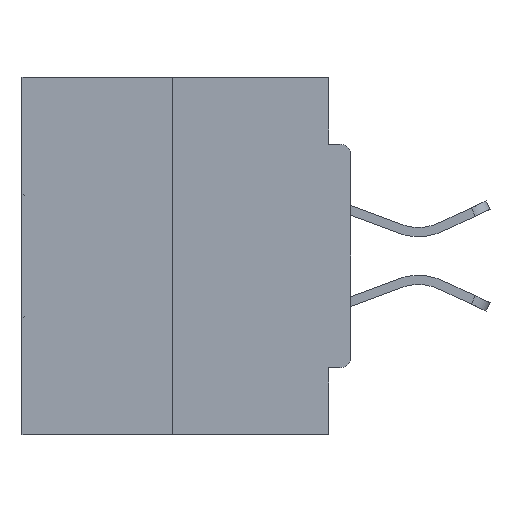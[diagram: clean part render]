
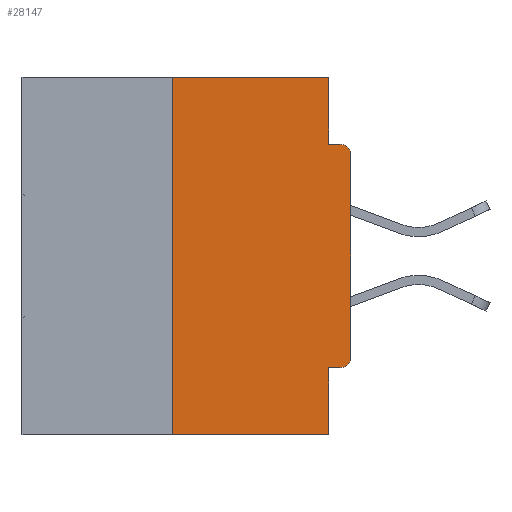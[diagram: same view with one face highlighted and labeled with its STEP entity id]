
A CAD part, left-side view. The second image highlights one B-rep face of the part: STEP entity #28147.
In plain terms, the highlighted planar face has unit normal (-1, 0, 0).
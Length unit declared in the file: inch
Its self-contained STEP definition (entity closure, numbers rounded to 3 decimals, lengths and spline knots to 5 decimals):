
#302 = EDGE_CURVE ( 'NONE', #27543, #3065, #4246, .T. ) ;
#587 = CARTESIAN_POINT ( 'NONE',  ( 0., 0.031, -0.5 ) ) ;
#1290 = CARTESIAN_POINT ( 'NONE',  ( 0., 0.015, -0.1085 ) ) ;
#1628 = DIRECTION ( 'NONE',  ( 1., 0., 0. ) ) ;
#2584 = CARTESIAN_POINT ( 'NONE',  ( 0., 0.25, 0. ) ) ;
#2604 = DIRECTION ( 'NONE',  ( 0., 0., -1. ) ) ;
#2662 = EDGE_CURVE ( 'NONE', #27543, #30808, #4565, .T. ) ;
#3065 = VERTEX_POINT ( 'NONE', #35761 ) ;
#3363 = VECTOR ( 'NONE', #21606, 39.37008 ) ;
#3924 = VECTOR ( 'NONE', #36852, 39.37008 ) ;
#3927 = ORIENTED_EDGE ( 'NONE', *, *, #38037, .F. ) ;
#3954 = ORIENTED_EDGE ( 'NONE', *, *, #16453, .F. ) ;
#4164 = DIRECTION ( 'NONE',  ( -1., 0., 0. ) ) ;
#4246 = CIRCLE ( 'NONE', #15293, 0.015 ) ;
#4565 = LINE ( 'NONE', #33325, #33715 ) ;
#4693 = CIRCLE ( 'NONE', #7941, 0.015 ) ;
#4710 = ORIENTED_EDGE ( 'NONE', *, *, #302, .T. ) ;
#4768 = CARTESIAN_POINT ( 'NONE',  ( 0., 0.031, -0.5 ) ) ;
#4777 = VERTEX_POINT ( 'NONE', #17695 ) ;
#5092 = CARTESIAN_POINT ( 'NONE',  ( 0., 0.031, 0. ) ) ;
#5784 = VERTEX_POINT ( 'NONE', #28572 ) ;
#6227 = CARTESIAN_POINT ( 'NONE',  ( 0., 0.015, -0.4065 ) ) ;
#7941 = AXIS2_PLACEMENT_3D ( 'NONE', #1290, #4164, #16374 ) ;
#8535 = LINE ( 'NONE', #5092, #16248 ) ;
#8718 = EDGE_CURVE ( 'NONE', #39990, #32900, #9581, .T. ) ;
#9581 = LINE ( 'NONE', #34098, #3363 ) ;
#10080 = VERTEX_POINT ( 'NONE', #19390 ) ;
#10758 = CARTESIAN_POINT ( 'NONE',  ( 0., 0.015, -0.3915 ) ) ;
#12666 = ORIENTED_EDGE ( 'NONE', *, *, #2662, .F. ) ;
#13094 = LINE ( 'NONE', #25967, #13631 ) ;
#13631 = VECTOR ( 'NONE', #26352, 39.37008 ) ;
#14060 = ORIENTED_EDGE ( 'NONE', *, *, #26409, .F. ) ;
#14444 = DIRECTION ( 'NONE',  ( 0., 0., -1. ) ) ;
#14796 = DIRECTION ( 'NONE',  ( 0., 0., 1. ) ) ;
#15293 = AXIS2_PLACEMENT_3D ( 'NONE', #10758, #35110, #2604 ) ;
#15648 = CARTESIAN_POINT ( 'NONE',  ( 0., 0.031, -0.4065 ) ) ;
#16178 = CARTESIAN_POINT ( 'NONE',  ( 0., 0.25, -0.5 ) ) ;
#16248 = VECTOR ( 'NONE', #24031, 39.37008 ) ;
#16374 = DIRECTION ( 'NONE',  ( 0., 0., -1. ) ) ;
#16453 = EDGE_CURVE ( 'NONE', #4777, #10080, #13094, .T. ) ;
#17695 = CARTESIAN_POINT ( 'NONE',  ( 0., 0.25, 0. ) ) ;
#17770 = DIRECTION ( 'NONE',  ( 0., 1., 0. ) ) ;
#17862 = ORIENTED_EDGE ( 'NONE', *, *, #8718, .T. ) ;
#18670 = DIRECTION ( 'NONE',  ( 0., 0., 1. ) ) ;
#18926 = VECTOR ( 'NONE', #14796, 39.37008 ) ;
#19390 = CARTESIAN_POINT ( 'NONE',  ( 0., 0.031, 0. ) ) ;
#19485 = VERTEX_POINT ( 'NONE', #22591 ) ;
#21397 = VERTEX_POINT ( 'NONE', #31590 ) ;
#21606 = DIRECTION ( 'NONE',  ( 0., -1., 0. ) ) ;
#22591 = CARTESIAN_POINT ( 'NONE',  ( 0., 0., -0.1085 ) ) ;
#22668 = EDGE_LOOP ( 'NONE', ( #3954, #3927, #17862, #29811, #12666, #4710, #29615, #37163, #14060, #36213 ) ) ;
#23782 = LINE ( 'NONE', #2584, #18926 ) ;
#24031 = DIRECTION ( 'NONE',  ( 0., 0., -1. ) ) ;
#24596 = VECTOR ( 'NONE', #18670, 39.37008 ) ;
#24619 = CARTESIAN_POINT ( 'NONE',  ( 0., 0., 0. ) ) ;
#25485 = DIRECTION ( 'NONE',  ( 0., 0., -1. ) ) ;
#25537 = EDGE_CURVE ( 'NONE', #10080, #21397, #8535, .T. ) ;
#25967 = CARTESIAN_POINT ( 'NONE',  ( 0., 0.46, 0. ) ) ;
#26352 = DIRECTION ( 'NONE',  ( 0., -1., 0. ) ) ;
#26409 = EDGE_CURVE ( 'NONE', #21397, #5784, #32957, .T. ) ;
#27543 = VERTEX_POINT ( 'NONE', #6227 ) ;
#28147 = ADVANCED_FACE ( 'NONE', ( #31664 ), #28578, .F. ) ;
#28572 = CARTESIAN_POINT ( 'NONE',  ( 0., 0.015, -0.0935 ) ) ;
#28578 = PLANE ( 'NONE',  #29380 ) ;
#29380 = AXIS2_PLACEMENT_3D ( 'NONE', #35947, #1628, #14444 ) ;
#29449 = VECTOR ( 'NONE', #25485, 39.37008 ) ;
#29615 = ORIENTED_EDGE ( 'NONE', *, *, #35760, .T. ) ;
#29811 = ORIENTED_EDGE ( 'NONE', *, *, #40299, .F. ) ;
#29867 = CARTESIAN_POINT ( 'NONE',  ( 0., 0., -0.0935 ) ) ;
#30659 = LINE ( 'NONE', #587, #29449 ) ;
#30808 = VERTEX_POINT ( 'NONE', #15648 ) ;
#31590 = CARTESIAN_POINT ( 'NONE',  ( 0., 0.031, -0.0935 ) ) ;
#31664 = FACE_OUTER_BOUND ( 'NONE', #22668, .T. ) ;
#32900 = VERTEX_POINT ( 'NONE', #4768 ) ;
#32957 = LINE ( 'NONE', #29867, #3924 ) ;
#33325 = CARTESIAN_POINT ( 'NONE',  ( 0., 0., -0.4065 ) ) ;
#33715 = VECTOR ( 'NONE', #17770, 39.37008 ) ;
#34098 = CARTESIAN_POINT ( 'NONE',  ( 0., 0.46, -0.5 ) ) ;
#35110 = DIRECTION ( 'NONE',  ( -1., 0., 0. ) ) ;
#35760 = EDGE_CURVE ( 'NONE', #3065, #19485, #37703, .T. ) ;
#35761 = CARTESIAN_POINT ( 'NONE',  ( 0., 0., -0.3915 ) ) ;
#35947 = CARTESIAN_POINT ( 'NONE',  ( 0., 0.46, 0. ) ) ;
#36213 = ORIENTED_EDGE ( 'NONE', *, *, #25537, .F. ) ;
#36852 = DIRECTION ( 'NONE',  ( 0., -1., 0. ) ) ;
#37163 = ORIENTED_EDGE ( 'NONE', *, *, #40002, .T. ) ;
#37703 = LINE ( 'NONE', #24619, #24596 ) ;
#38037 = EDGE_CURVE ( 'NONE', #39990, #4777, #23782, .T. ) ;
#39990 = VERTEX_POINT ( 'NONE', #16178 ) ;
#40002 = EDGE_CURVE ( 'NONE', #19485, #5784, #4693, .T. ) ;
#40299 = EDGE_CURVE ( 'NONE', #30808, #32900, #30659, .T. ) ;
